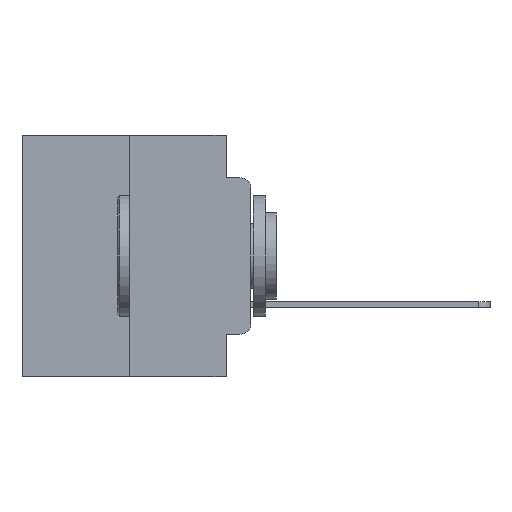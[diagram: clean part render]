
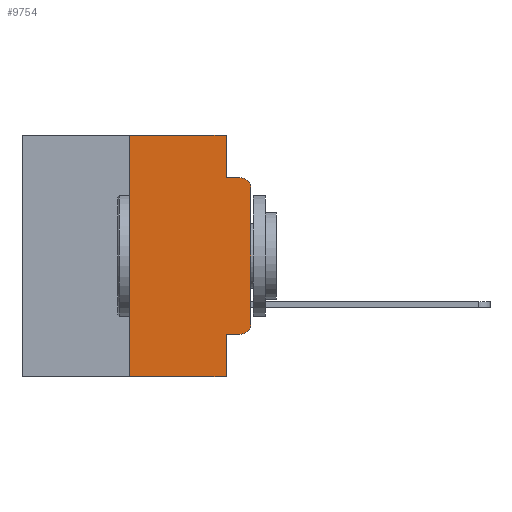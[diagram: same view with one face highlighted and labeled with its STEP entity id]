
A CAD part, left-side view. The second image highlights one B-rep face of the part: STEP entity #9754.
In plain terms, the highlighted planar face has unit normal (-1, 0, 0).
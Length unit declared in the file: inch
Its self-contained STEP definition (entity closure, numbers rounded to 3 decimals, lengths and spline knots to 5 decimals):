
#11 = CARTESIAN_POINT ( 'NONE',  ( 0., 0.473, 0. ) ) ;
#655 = CIRCLE ( 'NONE', #10551, 0.02 ) ;
#1032 = EDGE_CURVE ( 'NONE', #19156, #13721, #24173, .T. ) ;
#1077 = EDGE_CURVE ( 'NONE', #13721, #16341, #22903, .T. ) ;
#1114 = EDGE_CURVE ( 'NONE', #19466, #16341, #26876, .T. ) ;
#1291 = EDGE_CURVE ( 'NONE', #19475, #19466, #7085, .T. ) ;
#1329 = EDGE_CURVE ( 'NONE', #19955, #6279, #12261, .T. ) ;
#1423 = EDGE_CURVE ( 'NONE', #12385, #9709, #9596, .T. ) ;
#1459 = EDGE_CURVE ( 'NONE', #12385, #22159, #18736, .T. ) ;
#1505 = EDGE_CURVE ( 'NONE', #22159, #19156, #655, .T. ) ;
#1520 = EDGE_LOOP ( 'NONE', ( #2994, #16047, #26742, #23415, #19266, #25861, #14774, #16075, #5193, #12490 ) ) ;
#1565 = EDGE_CURVE ( 'NONE', #19955, #9709, #26265, .T. ) ;
#1914 = EDGE_CURVE ( 'NONE', #6279, #19475, #18084, .T. ) ;
#2351 = PLANE ( 'NONE',  #21384 ) ;
#2994 = ORIENTED_EDGE ( 'NONE', *, *, #1032, .T. ) ;
#3079 = CARTESIAN_POINT ( 'NONE',  ( 0., 0.25, 0. ) ) ;
#3926 = CARTESIAN_POINT ( 'NONE',  ( 0., 0.051, -0.5 ) ) ;
#4328 = FACE_OUTER_BOUND ( 'NONE', #1520, .T. ) ;
#4567 = VECTOR ( 'NONE', #5687, 39.37008 ) ;
#5023 = DIRECTION ( 'NONE',  ( 0., 0., 1. ) ) ;
#5168 = CARTESIAN_POINT ( 'NONE',  ( 0., 0.051, -0.4115 ) ) ;
#5193 = ORIENTED_EDGE ( 'NONE', *, *, #1459, .T. ) ;
#5217 = CARTESIAN_POINT ( 'NONE',  ( 0., 0.051, 0. ) ) ;
#5687 = DIRECTION ( 'NONE',  ( 0., -1., 0. ) ) ;
#6279 = VERTEX_POINT ( 'NONE', #3079 ) ;
#6336 = VECTOR ( 'NONE', #26152, 39.37008 ) ;
#7085 = LINE ( 'NONE', #5217, #6336 ) ;
#7106 = CARTESIAN_POINT ( 'NONE',  ( 0., 0.051, 0. ) ) ;
#7476 = VECTOR ( 'NONE', #5023, 39.37008 ) ;
#8211 = CARTESIAN_POINT ( 'NONE',  ( 0., 0.02, -0.1085 ) ) ;
#9249 = DIRECTION ( 'NONE',  ( 1., 0., 0. ) ) ;
#9596 = LINE ( 'NONE', #7106, #20003 ) ;
#9709 = VERTEX_POINT ( 'NONE', #3926 ) ;
#9754 = ADVANCED_FACE ( 'NONE', ( #4328 ), #2351, .F. ) ;
#10518 = CARTESIAN_POINT ( 'NONE',  ( 0., 0.25, -0.5 ) ) ;
#10551 = AXIS2_PLACEMENT_3D ( 'NONE', #21640, #25611, #20241 ) ;
#10640 = VECTOR ( 'NONE', #24423, 39.37008 ) ;
#11841 = DIRECTION ( 'NONE',  ( 0., 0., 1. ) ) ;
#12261 = LINE ( 'NONE', #17526, #27184 ) ;
#12385 = VERTEX_POINT ( 'NONE', #5168 ) ;
#12392 = CARTESIAN_POINT ( 'NONE',  ( 0., 0.473, 0. ) ) ;
#12490 = ORIENTED_EDGE ( 'NONE', *, *, #1505, .T. ) ;
#13236 = VECTOR ( 'NONE', #21200, 39.37008 ) ;
#13721 = VERTEX_POINT ( 'NONE', #16133 ) ;
#14206 = CARTESIAN_POINT ( 'NONE',  ( 0., 0., -0.3915 ) ) ;
#14774 = ORIENTED_EDGE ( 'NONE', *, *, #1565, .T. ) ;
#16047 = ORIENTED_EDGE ( 'NONE', *, *, #1077, .T. ) ;
#16075 = ORIENTED_EDGE ( 'NONE', *, *, #1423, .F. ) ;
#16133 = CARTESIAN_POINT ( 'NONE',  ( 0., 0., -0.1085 ) ) ;
#16239 = CARTESIAN_POINT ( 'NONE',  ( 0., 0.051, -0.0885 ) ) ;
#16341 = VERTEX_POINT ( 'NONE', #17285 ) ;
#16648 = AXIS2_PLACEMENT_3D ( 'NONE', #8211, #20770, #22826 ) ;
#17285 = CARTESIAN_POINT ( 'NONE',  ( 0., 0.02, -0.0885 ) ) ;
#17362 = CARTESIAN_POINT ( 'NONE',  ( 0., 0.051, -0.0885 ) ) ;
#17377 = CARTESIAN_POINT ( 'NONE',  ( 0., 0.051, -0.4115 ) ) ;
#17526 = CARTESIAN_POINT ( 'NONE',  ( 0., 0.25, 0. ) ) ;
#17764 = DIRECTION ( 'NONE',  ( 0., 0., -1. ) ) ;
#18084 = LINE ( 'NONE', #12392, #22228 ) ;
#18130 = DIRECTION ( 'NONE',  ( 0., -1., 0. ) ) ;
#18736 = LINE ( 'NONE', #17377, #13236 ) ;
#19156 = VERTEX_POINT ( 'NONE', #14206 ) ;
#19266 = ORIENTED_EDGE ( 'NONE', *, *, #1914, .F. ) ;
#19466 = VERTEX_POINT ( 'NONE', #17362 ) ;
#19475 = VERTEX_POINT ( 'NONE', #23534 ) ;
#19955 = VERTEX_POINT ( 'NONE', #10518 ) ;
#20003 = VECTOR ( 'NONE', #17764, 39.37008 ) ;
#20241 = DIRECTION ( 'NONE',  ( 0., 0., -1. ) ) ;
#20595 = CARTESIAN_POINT ( 'NONE',  ( 0., 0.473, -0.5 ) ) ;
#20770 = DIRECTION ( 'NONE',  ( -1., 0., 0. ) ) ;
#21200 = DIRECTION ( 'NONE',  ( 0., -1., 0. ) ) ;
#21384 = AXIS2_PLACEMENT_3D ( 'NONE', #11, #9249, #23771 ) ;
#21399 = CARTESIAN_POINT ( 'NONE',  ( 0., 0.02, -0.4115 ) ) ;
#21640 = CARTESIAN_POINT ( 'NONE',  ( 0., 0.02, -0.3915 ) ) ;
#21788 = CARTESIAN_POINT ( 'NONE',  ( 0., 0., 0. ) ) ;
#22159 = VERTEX_POINT ( 'NONE', #21399 ) ;
#22228 = VECTOR ( 'NONE', #18130, 39.37008 ) ;
#22826 = DIRECTION ( 'NONE',  ( 0., 0., -1. ) ) ;
#22903 = CIRCLE ( 'NONE', #16648, 0.02 ) ;
#23415 = ORIENTED_EDGE ( 'NONE', *, *, #1291, .F. ) ;
#23534 = CARTESIAN_POINT ( 'NONE',  ( 0., 0.051, 0. ) ) ;
#23771 = DIRECTION ( 'NONE',  ( 0., 0., -1. ) ) ;
#24173 = LINE ( 'NONE', #21788, #7476 ) ;
#24423 = DIRECTION ( 'NONE',  ( 0., -1., 0. ) ) ;
#25611 = DIRECTION ( 'NONE',  ( -1., 0., 0. ) ) ;
#25861 = ORIENTED_EDGE ( 'NONE', *, *, #1329, .F. ) ;
#26152 = DIRECTION ( 'NONE',  ( 0., 0., -1. ) ) ;
#26265 = LINE ( 'NONE', #20595, #4567 ) ;
#26742 = ORIENTED_EDGE ( 'NONE', *, *, #1114, .F. ) ;
#26876 = LINE ( 'NONE', #16239, #10640 ) ;
#27184 = VECTOR ( 'NONE', #11841, 39.37008 ) ;
